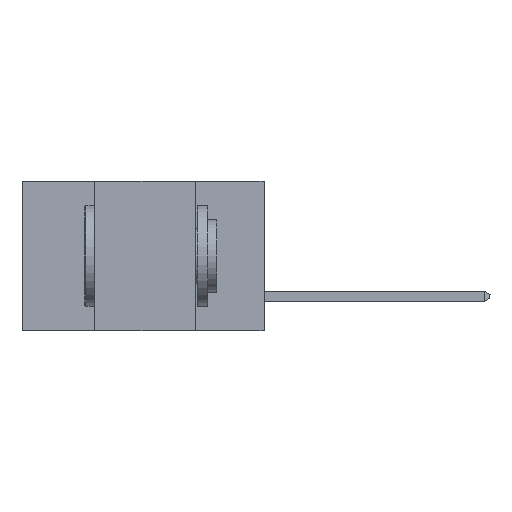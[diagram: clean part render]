
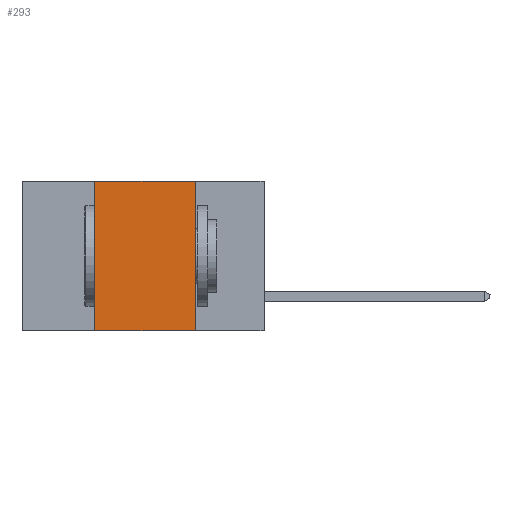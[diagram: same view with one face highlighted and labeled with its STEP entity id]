
A CAD part, left-side view. The second image highlights one B-rep face of the part: STEP entity #293.
In plain terms, the highlighted planar face has unit normal (-1, 0, 0).
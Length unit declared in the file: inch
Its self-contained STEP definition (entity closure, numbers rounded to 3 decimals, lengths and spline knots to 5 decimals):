
#292 = EDGE_CURVE ( 'NONE', #9451, #4834, #11030, .T. ) ;
#293 = ADVANCED_FACE ( 'NONE', ( #10972 ), #2605, .F. ) ;
#1094 = CARTESIAN_POINT ( 'NONE',  ( 0., 0.17, -0.37 ) ) ;
#1529 = VERTEX_POINT ( 'NONE', #3317 ) ;
#2095 = EDGE_LOOP ( 'NONE', ( #4095, #5439, #10728, #2686 ) ) ;
#2431 = LINE ( 'NONE', #10726, #10809 ) ;
#2605 = PLANE ( 'NONE',  #11187 ) ;
#2663 = CARTESIAN_POINT ( 'NONE',  ( 0., 0.6, -0.37 ) ) ;
#2686 = ORIENTED_EDGE ( 'NONE', *, *, #292, .T. ) ;
#3141 = EDGE_CURVE ( 'NONE', #11491, #1529, #6316, .T. ) ;
#3317 = CARTESIAN_POINT ( 'NONE',  ( 0., 0.17, 0. ) ) ;
#4095 = ORIENTED_EDGE ( 'NONE', *, *, #8297, .F. ) ;
#4341 = DIRECTION ( 'NONE',  ( 1., 0., 0. ) ) ;
#4489 = DIRECTION ( 'NONE',  ( 0., -1., 0. ) ) ;
#4834 = VERTEX_POINT ( 'NONE', #1094 ) ;
#5317 = CARTESIAN_POINT ( 'NONE',  ( 0., 0.6, 0. ) ) ;
#5439 = ORIENTED_EDGE ( 'NONE', *, *, #3141, .F. ) ;
#6064 = CARTESIAN_POINT ( 'NONE',  ( 0., 0.42, 0. ) ) ;
#6316 = LINE ( 'NONE', #8187, #11512 ) ;
#7241 = DIRECTION ( 'NONE',  ( 0., 0., 1. ) ) ;
#7414 = CARTESIAN_POINT ( 'NONE',  ( 0., 0.42, -0.37 ) ) ;
#7486 = LINE ( 'NONE', #7414, #8295 ) ;
#7699 = CARTESIAN_POINT ( 'NONE',  ( 0., 0.42, -0.37 ) ) ;
#8187 = CARTESIAN_POINT ( 'NONE',  ( 0., 0.6, 0. ) ) ;
#8295 = VECTOR ( 'NONE', #7241, 39.37008 ) ;
#8297 = EDGE_CURVE ( 'NONE', #1529, #4834, #2431, .T. ) ;
#9125 = DIRECTION ( 'NONE',  ( 0., 0., -1. ) ) ;
#9451 = VERTEX_POINT ( 'NONE', #7699 ) ;
#10726 = CARTESIAN_POINT ( 'NONE',  ( 0., 0.17, -0.37 ) ) ;
#10728 = ORIENTED_EDGE ( 'NONE', *, *, #11977, .F. ) ;
#10809 = VECTOR ( 'NONE', #10915, 39.37008 ) ;
#10908 = DIRECTION ( 'NONE',  ( 0., -1., 0. ) ) ;
#10915 = DIRECTION ( 'NONE',  ( 0., 0., -1. ) ) ;
#10972 = FACE_OUTER_BOUND ( 'NONE', #2095, .T. ) ;
#11030 = LINE ( 'NONE', #2663, #11942 ) ;
#11187 = AXIS2_PLACEMENT_3D ( 'NONE', #5317, #4341, #9125 ) ;
#11491 = VERTEX_POINT ( 'NONE', #6064 ) ;
#11512 = VECTOR ( 'NONE', #4489, 39.37008 ) ;
#11942 = VECTOR ( 'NONE', #10908, 39.37008 ) ;
#11977 = EDGE_CURVE ( 'NONE', #9451, #11491, #7486, .T. ) ;
